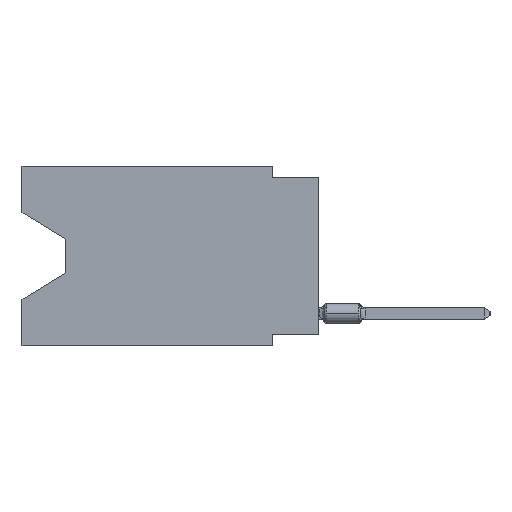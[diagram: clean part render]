
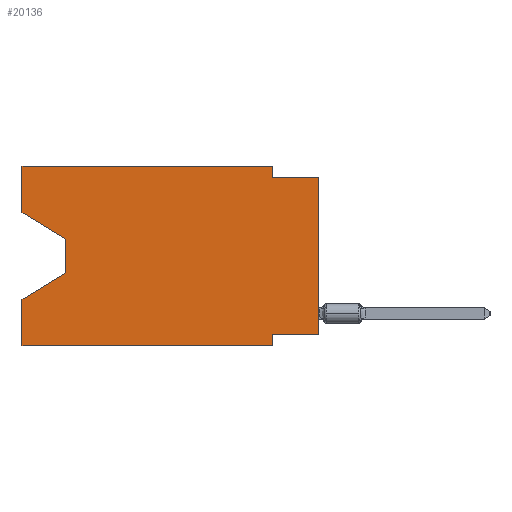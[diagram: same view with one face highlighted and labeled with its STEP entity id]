
A CAD part, left-side view. The second image highlights one B-rep face of the part: STEP entity #20136.
In plain terms, the highlighted planar face has unit normal (-1, 0, 0).
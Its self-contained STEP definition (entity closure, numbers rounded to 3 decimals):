
#493 = EDGE_CURVE ( 'NONE', #61849, #61379, #34345, .T. ) ;
#1028 = VERTEX_POINT ( 'NONE', #36721 ) ;
#1318 = CARTESIAN_POINT ( 'NONE',  ( 0., 16.383, 0. ) ) ;
#2165 = EDGE_CURVE ( 'NONE', #44420, #56616, #26078, .T. ) ;
#2445 = LINE ( 'NONE', #46730, #56788 ) ;
#2783 = EDGE_CURVE ( 'NONE', #5772, #10458, #7449, .T. ) ;
#3476 = PLANE ( 'NONE',  #61477 ) ;
#5116 = CARTESIAN_POINT ( 'NONE',  ( 0., 16.383, 0. ) ) ;
#5564 = VERTEX_POINT ( 'NONE', #7467 ) ;
#5772 = VERTEX_POINT ( 'NONE', #10647 ) ;
#5784 = EDGE_CURVE ( 'NONE', #44420, #13345, #15162, .T. ) ;
#6558 = CARTESIAN_POINT ( 'NONE',  ( 0., 2.54, -9.906 ) ) ;
#6716 = VECTOR ( 'NONE', #49908, 1000. ) ;
#7164 = VECTOR ( 'NONE', #10963, 1000. ) ;
#7449 = LINE ( 'NONE', #32190, #17158 ) ;
#7467 = CARTESIAN_POINT ( 'NONE',  ( 0., 0., -9.271 ) ) ;
#8144 = LINE ( 'NONE', #22283, #17508 ) ;
#8956 = CARTESIAN_POINT ( 'NONE',  ( 0., 13.97, -4.013 ) ) ;
#9460 = LINE ( 'NONE', #24868, #6716 ) ;
#9930 = ORIENTED_EDGE ( 'NONE', *, *, #45024, .F. ) ;
#10458 = VERTEX_POINT ( 'NONE', #63499 ) ;
#10570 = CARTESIAN_POINT ( 'NONE',  ( 0., 0., -0.635 ) ) ;
#10647 = CARTESIAN_POINT ( 'NONE',  ( 0., 2.54, 0. ) ) ;
#10753 = EDGE_CURVE ( 'NONE', #5564, #1028, #2445, .T. ) ;
#10963 = DIRECTION ( 'NONE',  ( 0., -1., 0. ) ) ;
#11023 = EDGE_CURVE ( 'NONE', #36459, #26117, #16773, .T. ) ;
#12543 = DIRECTION ( 'NONE',  ( 0., 0., 1. ) ) ;
#12656 = DIRECTION ( 'NONE',  ( 0., -1., 0. ) ) ;
#13345 = VERTEX_POINT ( 'NONE', #6558 ) ;
#13429 = FACE_OUTER_BOUND ( 'NONE', #58873, .T. ) ;
#14438 = CARTESIAN_POINT ( 'NONE',  ( 0., 16.383, -2.546 ) ) ;
#15162 = LINE ( 'NONE', #30883, #7164 ) ;
#16773 = LINE ( 'NONE', #31529, #61927 ) ;
#17158 = VECTOR ( 'NONE', #56903, 1000. ) ;
#17394 = DIRECTION ( 'NONE',  ( 0., 0., -1. ) ) ;
#17508 = VECTOR ( 'NONE', #12656, 1000. ) ;
#18119 = DIRECTION ( 'NONE',  ( 0., 0., -1. ) ) ;
#18614 = DIRECTION ( 'NONE',  ( 0., -0.855, -0.519 ) ) ;
#20136 = ADVANCED_FACE ( 'NONE', ( #13429 ), #3476, .F. ) ;
#22029 = DIRECTION ( 'NONE',  ( 0., 1., 0. ) ) ;
#22098 = DIRECTION ( 'NONE',  ( 0., 0., -1. ) ) ;
#22283 = CARTESIAN_POINT ( 'NONE',  ( 0., 16.383, 0. ) ) ;
#24716 = LINE ( 'NONE', #44295, #46116 ) ;
#24868 = CARTESIAN_POINT ( 'NONE',  ( 0., 13.97, -5.893 ) ) ;
#24896 = ORIENTED_EDGE ( 'NONE', *, *, #58576, .F. ) ;
#25174 = ORIENTED_EDGE ( 'NONE', *, *, #493, .F. ) ;
#26078 = LINE ( 'NONE', #60433, #49892 ) ;
#26117 = VERTEX_POINT ( 'NONE', #27572 ) ;
#27070 = CARTESIAN_POINT ( 'NONE',  ( 0., 16.383, -9.906 ) ) ;
#27090 = VECTOR ( 'NONE', #53948, 1000. ) ;
#27572 = CARTESIAN_POINT ( 'NONE',  ( 0., 13.97, -5.893 ) ) ;
#27841 = EDGE_CURVE ( 'NONE', #5564, #29066, #24716, .T. ) ;
#28551 = ORIENTED_EDGE ( 'NONE', *, *, #2783, .F. ) ;
#29066 = VERTEX_POINT ( 'NONE', #45298 ) ;
#30883 = CARTESIAN_POINT ( 'NONE',  ( 0., 16.383, -9.906 ) ) ;
#31529 = CARTESIAN_POINT ( 'NONE',  ( 0., 13.97, -4.013 ) ) ;
#32190 = CARTESIAN_POINT ( 'NONE',  ( 0., 2.54, 0. ) ) ;
#34345 = LINE ( 'NONE', #5116, #27090 ) ;
#34433 = ORIENTED_EDGE ( 'NONE', *, *, #57950, .T. ) ;
#34565 = VECTOR ( 'NONE', #50063, 1000. ) ;
#34980 = LINE ( 'NONE', #10570, #34565 ) ;
#36459 = VERTEX_POINT ( 'NONE', #8956 ) ;
#36721 = CARTESIAN_POINT ( 'NONE',  ( 0., 2.54, -9.271 ) ) ;
#37385 = LINE ( 'NONE', #56967, #62272 ) ;
#38682 = ORIENTED_EDGE ( 'NONE', *, *, #5784, .T. ) ;
#38735 = ORIENTED_EDGE ( 'NONE', *, *, #2165, .F. ) ;
#41393 = ORIENTED_EDGE ( 'NONE', *, *, #56265, .T. ) ;
#42645 = CARTESIAN_POINT ( 'NONE',  ( 0., 16.383, 0. ) ) ;
#42849 = ORIENTED_EDGE ( 'NONE', *, *, #62774, .F. ) ;
#44295 = CARTESIAN_POINT ( 'NONE',  ( 0., 0., 0. ) ) ;
#44420 = VERTEX_POINT ( 'NONE', #27070 ) ;
#45024 = EDGE_CURVE ( 'NONE', #10458, #29066, #34980, .T. ) ;
#45298 = CARTESIAN_POINT ( 'NONE',  ( 0., 0., -0.635 ) ) ;
#46050 = ORIENTED_EDGE ( 'NONE', *, *, #27841, .T. ) ;
#46116 = VECTOR ( 'NONE', #59076, 1000. ) ;
#46730 = CARTESIAN_POINT ( 'NONE',  ( 0., 0., -9.271 ) ) ;
#49892 = VECTOR ( 'NONE', #12543, 1000. ) ;
#49908 = DIRECTION ( 'NONE',  ( 0., 0.855, -0.519 ) ) ;
#49948 = ORIENTED_EDGE ( 'NONE', *, *, #10753, .F. ) ;
#50063 = DIRECTION ( 'NONE',  ( 0., -1., 0. ) ) ;
#52316 = CARTESIAN_POINT ( 'NONE',  ( 0., 16.383, -7.36 ) ) ;
#53948 = DIRECTION ( 'NONE',  ( 0., 0., 1. ) ) ;
#56039 = ORIENTED_EDGE ( 'NONE', *, *, #11023, .T. ) ;
#56103 = CARTESIAN_POINT ( 'NONE',  ( 0., 16.383, -2.546 ) ) ;
#56139 = DIRECTION ( 'NONE',  ( 1., 0., 0. ) ) ;
#56265 = EDGE_CURVE ( 'NONE', #26117, #56616, #9460, .T. ) ;
#56616 = VERTEX_POINT ( 'NONE', #52316 ) ;
#56788 = VECTOR ( 'NONE', #22029, 1000. ) ;
#56903 = DIRECTION ( 'NONE',  ( 0., 0., -1. ) ) ;
#56967 = CARTESIAN_POINT ( 'NONE',  ( 0., 2.54, -9.906 ) ) ;
#57950 = EDGE_CURVE ( 'NONE', #61849, #36459, #62609, .T. ) ;
#58576 = EDGE_CURVE ( 'NONE', #1028, #13345, #37385, .T. ) ;
#58873 = EDGE_LOOP ( 'NONE', ( #34433, #56039, #41393, #38735, #38682, #24896, #49948, #46050, #9930, #28551, #42849, #25174 ) ) ;
#59076 = DIRECTION ( 'NONE',  ( 0., 0., 1. ) ) ;
#60433 = CARTESIAN_POINT ( 'NONE',  ( 0., 16.383, 0. ) ) ;
#61206 = VECTOR ( 'NONE', #18614, 1000. ) ;
#61379 = VERTEX_POINT ( 'NONE', #1318 ) ;
#61477 = AXIS2_PLACEMENT_3D ( 'NONE', #42645, #56139, #22098 ) ;
#61849 = VERTEX_POINT ( 'NONE', #56103 ) ;
#61927 = VECTOR ( 'NONE', #17394, 1000. ) ;
#62272 = VECTOR ( 'NONE', #18119, 1000. ) ;
#62609 = LINE ( 'NONE', #14438, #61206 ) ;
#62774 = EDGE_CURVE ( 'NONE', #61379, #5772, #8144, .T. ) ;
#63499 = CARTESIAN_POINT ( 'NONE',  ( 0., 2.54, -0.635 ) ) ;
